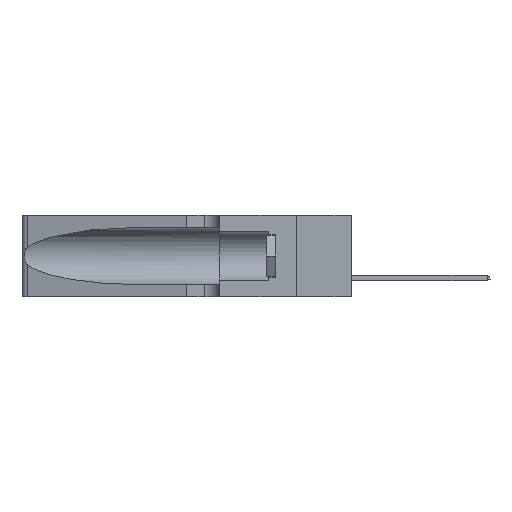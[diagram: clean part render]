
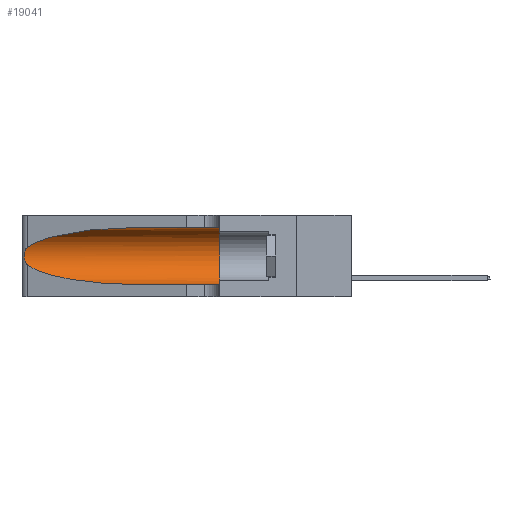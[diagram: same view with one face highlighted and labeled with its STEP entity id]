
A CAD part, left-side view. The second image highlights one B-rep face of the part: STEP entity #19041.
In plain terms, the highlighted cylindrical face has radius 3.308 mm (diameter 6.617 mm), a partial arc.
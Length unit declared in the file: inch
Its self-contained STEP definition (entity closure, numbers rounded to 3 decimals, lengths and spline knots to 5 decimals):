
#327 = CARTESIAN_POINT ( 'NONE',  ( 0.1305, 1.61858, 0.185 ) ) ;
#650 = CARTESIAN_POINT ( 'NONE',  ( 0.26075, 1.23896, 0.19203 ) ) ;
#692 = ORIENTED_EDGE ( 'NONE', *, *, #20325, .T. ) ;
#1034 = CARTESIAN_POINT ( 'NONE',  ( 0.25555, 1.22994, 0.2215 ) ) ;
#1053 = VERTEX_POINT ( 'NONE', #15738 ) ;
#1559 = AXIS2_PLACEMENT_3D ( 'NONE', #12219, #21162, #16348 ) ;
#2180 = CARTESIAN_POINT ( 'NONE',  ( 0.18966, 0.96281, 0.31525 ) ) ;
#3901 = CARTESIAN_POINT ( 'NONE',  ( 0.1305, 1.61858, 0.05475 ) ) ;
#4209 = CYLINDRICAL_SURFACE ( 'NONE', #13514, 0.13025 ) ;
#4289 = ORIENTED_EDGE ( 'NONE', *, *, #19009, .T. ) ;
#4662 = ORIENTED_EDGE ( 'NONE', *, *, #18673, .F. ) ;
#5431 = CARTESIAN_POINT ( 'NONE',  ( 0.2373, 1.15595, 0.08982 ) ) ;
#6764 = VERTEX_POINT ( 'NONE', #17740 ) ;
#6827 = DIRECTION ( 'NONE',  ( 0., -1., 0. ) ) ;
#7367 = CARTESIAN_POINT ( 'NONE',  ( 0.18966, 0.96281, 0.05475 ) ) ;
#7465 = CARTESIAN_POINT ( 'NONE',  ( 0.25487, 1.22718, 0.14631 ) ) ;
#7886 = CARTESIAN_POINT ( 'NONE',  ( 0.1305, 0.72297, 0.05475 ) ) ;
#9381 = VERTEX_POINT ( 'NONE', #7886 ) ;
#9447 = CIRCLE ( 'NONE', #1559, 0.13025 ) ;
#9769 = FACE_OUTER_BOUND ( 'NONE', #11192, .T. ) ;
#9888 = CARTESIAN_POINT ( 'NONE',  ( 0.25487, 1.22718, 0.22369 ) ) ;
#10015 = EDGE_CURVE ( 'NONE', #21371, #1053, #11159, .T. ) ;
#10055 = EDGE_CURVE ( 'NONE', #9381, #6764, #23640, .T. ) ;
#10798 = VECTOR ( 'NONE', #6827, 39.37008 ) ;
#11159 = LINE ( 'NONE', #12656, #10798 ) ;
#11192 = EDGE_LOOP ( 'NONE', ( #4289, #692, #22944, #18090, #4662, #16325 ) ) ;
#11497 = VERTEX_POINT ( 'NONE', #18828 ) ;
#11753 = CARTESIAN_POINT ( 'NONE',  ( 0.26075, 1.23896, 0.178 ) ) ;
#11844 = CARTESIAN_POINT ( 'NONE',  ( 0.26018, 1.23835, 0.19895 ) ) ;
#11939 = CARTESIAN_POINT ( 'NONE',  ( 0.25789, 1.23486, 0.15765 ) ) ;
#12104 = CARTESIAN_POINT ( 'NONE',  ( 0.1305, 0.72297, 0.31525 ) ) ;
#12122 = CARTESIAN_POINT ( 'NONE',  ( 0.25487, 1.22718, 0.14631 ) ) ;
#12219 = CARTESIAN_POINT ( 'NONE',  ( 0.1305, 0.35, 0.185 ) ) ;
#12508 = B_SPLINE_CURVE_WITH_KNOTS ( 'NONE', 3,
 ( #9888, #1034, #25440, #25341, #16444, #11844, #650, #11753, #27420, #14093, #11939, #18757, #23110, #12122 ),
 .UNSPECIFIED., .F., .F.,
 ( 4, 2, 2, 2, 2, 2, 4 ),
 ( 0., 0.00027, 0.00053, 0.00107, 0.0016, 0.00187, 0.00214 ),
 .UNSPECIFIED. ) ;
#12656 = CARTESIAN_POINT ( 'NONE',  ( 0.1305, 1.61858, 0.31525 ) ) ;
#13514 = AXIS2_PLACEMENT_3D ( 'NONE', #327, #27395, #15558 ) ;
#14093 = CARTESIAN_POINT ( 'NONE',  ( 0.25856, 1.23593, 0.16098 ) ) ;
#15550 = EDGE_CURVE ( 'NONE', #11497, #9381, #16648, .T. ) ;
#15558 = DIRECTION ( 'NONE',  ( 0., 0., -1. ) ) ;
#15738 = CARTESIAN_POINT ( 'NONE',  ( 0.1305, 0.35, 0.31525 ) ) ;
#15844 = CARTESIAN_POINT ( 'NONE',  ( 0.2373, 1.15595, 0.28018 ) ) ;
#16262 = CARTESIAN_POINT ( 'NONE',  ( 0.1305, 0.72297, 0.05475 ) ) ;
#16325 = ORIENTED_EDGE ( 'NONE', *, *, #10015, .F. ) ;
#16348 = DIRECTION ( 'NONE',  ( 0., 0., 1. ) ) ;
#16444 = CARTESIAN_POINT ( 'NONE',  ( 0.25854, 1.2359, 0.20912 ) ) ;
#16648 =( BOUNDED_CURVE ( )  B_SPLINE_CURVE ( 3, ( #7465, #5431, #7367, #16262 ),
 .UNSPECIFIED., .F., .T. ) 
 B_SPLINE_CURVE_WITH_KNOTS ( ( 4, 4 ),
 ( 3.44316, 4.71239 ),
 .UNSPECIFIED. ) 
 CURVE ( )  GEOMETRIC_REPRESENTATION_ITEM ( )  RATIONAL_B_SPLINE_CURVE ( ( 1., 0.87, 0.87, 1. ) ) 
 REPRESENTATION_ITEM ( '' )  );
#17715 =( BOUNDED_CURVE ( )  B_SPLINE_CURVE ( 3, ( #20180, #2180, #15844, #17972 ),
 .UNSPECIFIED., .F., .T. ) 
 B_SPLINE_CURVE_WITH_KNOTS ( ( 4, 4 ),
 ( 1.5708, 2.84003 ),
 .UNSPECIFIED. ) 
 CURVE ( )  GEOMETRIC_REPRESENTATION_ITEM ( )  RATIONAL_B_SPLINE_CURVE ( ( 1., 0.87, 0.87, 1. ) ) 
 REPRESENTATION_ITEM ( '' )  );
#17740 = CARTESIAN_POINT ( 'NONE',  ( 0.1305, 0.35, 0.05475 ) ) ;
#17972 = CARTESIAN_POINT ( 'NONE',  ( 0.25487, 1.22718, 0.22369 ) ) ;
#18090 = ORIENTED_EDGE ( 'NONE', *, *, #10055, .T. ) ;
#18673 = EDGE_CURVE ( 'NONE', #1053, #6764, #9447, .T. ) ;
#18757 = CARTESIAN_POINT ( 'NONE',  ( 0.25639, 1.23186, 0.15144 ) ) ;
#18828 = CARTESIAN_POINT ( 'NONE',  ( 0.25487, 1.22718, 0.14631 ) ) ;
#19009 = EDGE_CURVE ( 'NONE', #21371, #24189, #17715, .T. ) ;
#19041 = ADVANCED_FACE ( 'NONE', ( #9769 ), #4209, .F. ) ;
#20180 = CARTESIAN_POINT ( 'NONE',  ( 0.1305, 0.72297, 0.31525 ) ) ;
#20325 = EDGE_CURVE ( 'NONE', #24189, #11497, #12508, .T. ) ;
#20336 = DIRECTION ( 'NONE',  ( 0., -1., 0. ) ) ;
#21162 = DIRECTION ( 'NONE',  ( 0., 1., 0. ) ) ;
#21371 = VERTEX_POINT ( 'NONE', #12104 ) ;
#22944 = ORIENTED_EDGE ( 'NONE', *, *, #15550, .T. ) ;
#23110 = CARTESIAN_POINT ( 'NONE',  ( 0.25555, 1.22993, 0.14849 ) ) ;
#23640 = LINE ( 'NONE', #3901, #27158 ) ;
#24189 = VERTEX_POINT ( 'NONE', #27888 ) ;
#25341 = CARTESIAN_POINT ( 'NONE',  ( 0.25787, 1.23484, 0.2124 ) ) ;
#25440 = CARTESIAN_POINT ( 'NONE',  ( 0.25639, 1.23184, 0.21858 ) ) ;
#27158 = VECTOR ( 'NONE', #20336, 39.37008 ) ;
#27395 = DIRECTION ( 'NONE',  ( 0., -1., 0. ) ) ;
#27420 = CARTESIAN_POINT ( 'NONE',  ( 0.26017, 1.23833, 0.17102 ) ) ;
#27888 = CARTESIAN_POINT ( 'NONE',  ( 0.25487, 1.22718, 0.22369 ) ) ;
